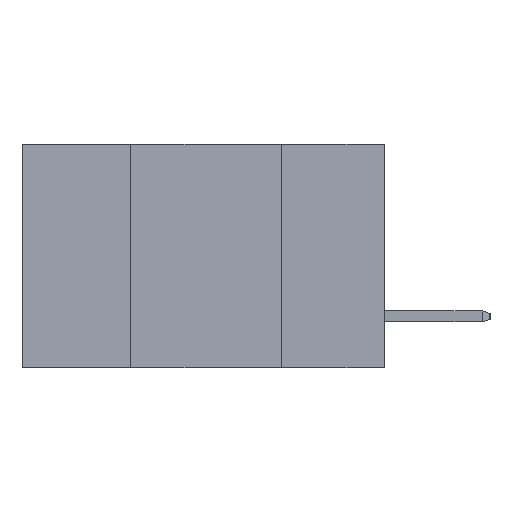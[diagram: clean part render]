
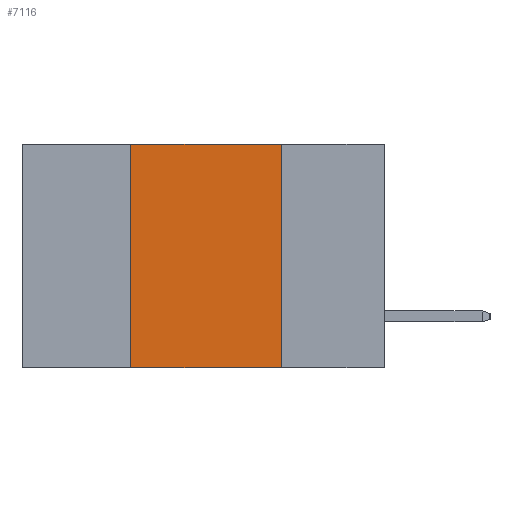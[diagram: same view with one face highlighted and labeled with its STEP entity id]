
A CAD part, left-side view. The second image highlights one B-rep face of the part: STEP entity #7116.
In plain terms, the highlighted planar face has unit normal (-1, 0, 0).
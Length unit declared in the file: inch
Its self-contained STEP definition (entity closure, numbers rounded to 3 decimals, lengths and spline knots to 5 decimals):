
#478 = VECTOR ( 'NONE', #7871, 39.37008 ) ;
#737 = CARTESIAN_POINT ( 'NONE',  ( 0., 0.17, 0. ) ) ;
#911 = VERTEX_POINT ( 'NONE', #10139 ) ;
#1657 = CARTESIAN_POINT ( 'NONE',  ( 0., 0.6, 0. ) ) ;
#1664 = VECTOR ( 'NONE', #3748, 39.37008 ) ;
#2186 = VERTEX_POINT ( 'NONE', #10461 ) ;
#2493 = DIRECTION ( 'NONE',  ( 0., 0., -1. ) ) ;
#2695 = LINE ( 'NONE', #9427, #478 ) ;
#2797 = CARTESIAN_POINT ( 'NONE',  ( 0., 0.42, 0. ) ) ;
#2867 = CARTESIAN_POINT ( 'NONE',  ( 0., 0.42, -0.37 ) ) ;
#3748 = DIRECTION ( 'NONE',  ( 0., -1., 0. ) ) ;
#4015 = DIRECTION ( 'NONE',  ( 0., 0., -1. ) ) ;
#4203 = EDGE_CURVE ( 'NONE', #10370, #911, #4216, .T. ) ;
#4216 = LINE ( 'NONE', #2797, #5931 ) ;
#4399 = ORIENTED_EDGE ( 'NONE', *, *, #8657, .F. ) ;
#4518 = ORIENTED_EDGE ( 'NONE', *, *, #9241, .T. ) ;
#4578 = VECTOR ( 'NONE', #4015, 39.37008 ) ;
#5453 = VERTEX_POINT ( 'NONE', #6070 ) ;
#5513 = LINE ( 'NONE', #6986, #1664 ) ;
#5931 = VECTOR ( 'NONE', #6457, 39.37008 ) ;
#6070 = CARTESIAN_POINT ( 'NONE',  ( 0., 0.17, -0.37 ) ) ;
#6457 = DIRECTION ( 'NONE',  ( 0., 0., 1. ) ) ;
#6559 = LINE ( 'NONE', #737, #4578 ) ;
#6566 = PLANE ( 'NONE',  #8017 ) ;
#6986 = CARTESIAN_POINT ( 'NONE',  ( 0., 0.6, -0.37 ) ) ;
#7116 = ADVANCED_FACE ( 'NONE', ( #8074 ), #6566, .F. ) ;
#7350 = ORIENTED_EDGE ( 'NONE', *, *, #4203, .F. ) ;
#7378 = DIRECTION ( 'NONE',  ( 1., 0., 0. ) ) ;
#7446 = ORIENTED_EDGE ( 'NONE', *, *, #7680, .F. ) ;
#7680 = EDGE_CURVE ( 'NONE', #2186, #5453, #6559, .T. ) ;
#7871 = DIRECTION ( 'NONE',  ( 0., -1., 0. ) ) ;
#8017 = AXIS2_PLACEMENT_3D ( 'NONE', #1657, #7378, #2493 ) ;
#8074 = FACE_OUTER_BOUND ( 'NONE', #8161, .T. ) ;
#8161 = EDGE_LOOP ( 'NONE', ( #7446, #4399, #7350, #4518 ) ) ;
#8657 = EDGE_CURVE ( 'NONE', #911, #2186, #2695, .T. ) ;
#9241 = EDGE_CURVE ( 'NONE', #10370, #5453, #5513, .T. ) ;
#9427 = CARTESIAN_POINT ( 'NONE',  ( 0., 0.6, 0. ) ) ;
#10139 = CARTESIAN_POINT ( 'NONE',  ( 0., 0.42, 0. ) ) ;
#10370 = VERTEX_POINT ( 'NONE', #2867 ) ;
#10461 = CARTESIAN_POINT ( 'NONE',  ( 0., 0.17, 0. ) ) ;
